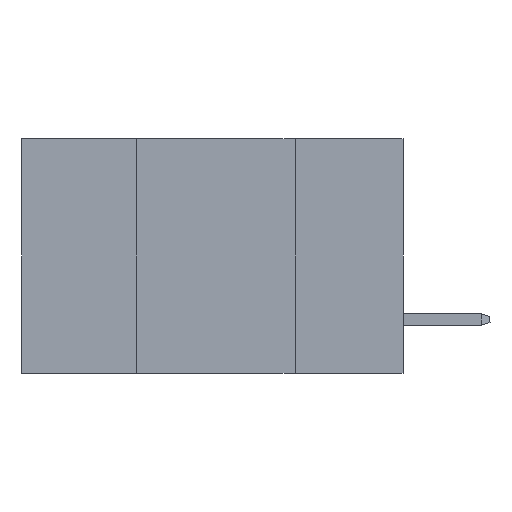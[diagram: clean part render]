
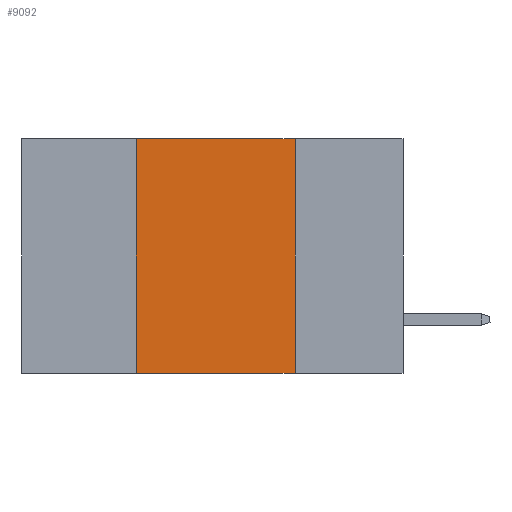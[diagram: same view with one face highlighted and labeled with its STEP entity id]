
A CAD part, left-side view. The second image highlights one B-rep face of the part: STEP entity #9092.
In plain terms, the highlighted planar face has unit normal (-1, 0, 0).
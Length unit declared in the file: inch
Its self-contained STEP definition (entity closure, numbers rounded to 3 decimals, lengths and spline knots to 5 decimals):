
#699 = VECTOR ( 'NONE', #11565, 39.37008 ) ;
#727 = EDGE_CURVE ( 'NONE', #1597, #11515, #3971, .T. ) ;
#1251 = EDGE_CURVE ( 'NONE', #15855, #9012, #5913, .T. ) ;
#1597 = VERTEX_POINT ( 'NONE', #13618 ) ;
#1926 = VECTOR ( 'NONE', #8427, 39.37008 ) ;
#2162 = PLANE ( 'NONE',  #11635 ) ;
#3344 = LINE ( 'NONE', #14631, #1926 ) ;
#3499 = DIRECTION ( 'NONE',  ( 0., 0., -1. ) ) ;
#3557 = DIRECTION ( 'NONE',  ( 0., 0., -1. ) ) ;
#3971 = LINE ( 'NONE', #5391, #8766 ) ;
#5391 = CARTESIAN_POINT ( 'NONE',  ( 0., 0.42, 0. ) ) ;
#5913 = LINE ( 'NONE', #5993, #7078 ) ;
#5993 = CARTESIAN_POINT ( 'NONE',  ( 0., 0.17, 0. ) ) ;
#6064 = FACE_OUTER_BOUND ( 'NONE', #6516, .T. ) ;
#6501 = CARTESIAN_POINT ( 'NONE',  ( 0., 0.6, 0. ) ) ;
#6516 = EDGE_LOOP ( 'NONE', ( #11091, #13093, #14889, #9731 ) ) ;
#7078 = VECTOR ( 'NONE', #3499, 39.37008 ) ;
#7250 = EDGE_CURVE ( 'NONE', #11515, #15855, #8907, .T. ) ;
#7310 = CARTESIAN_POINT ( 'NONE',  ( 0., 0.6, 0. ) ) ;
#8427 = DIRECTION ( 'NONE',  ( 0., -1., 0. ) ) ;
#8766 = VECTOR ( 'NONE', #9043, 39.37008 ) ;
#8907 = LINE ( 'NONE', #6501, #699 ) ;
#9012 = VERTEX_POINT ( 'NONE', #10788 ) ;
#9043 = DIRECTION ( 'NONE',  ( 0., 0., 1. ) ) ;
#9092 = ADVANCED_FACE ( 'NONE', ( #6064 ), #2162, .F. ) ;
#9423 = CARTESIAN_POINT ( 'NONE',  ( 0., 0.17, 0. ) ) ;
#9731 = ORIENTED_EDGE ( 'NONE', *, *, #14027, .T. ) ;
#10788 = CARTESIAN_POINT ( 'NONE',  ( 0., 0.17, -0.37 ) ) ;
#11091 = ORIENTED_EDGE ( 'NONE', *, *, #1251, .F. ) ;
#11515 = VERTEX_POINT ( 'NONE', #13627 ) ;
#11565 = DIRECTION ( 'NONE',  ( 0., -1., 0. ) ) ;
#11635 = AXIS2_PLACEMENT_3D ( 'NONE', #7310, #13700, #3557 ) ;
#13093 = ORIENTED_EDGE ( 'NONE', *, *, #7250, .F. ) ;
#13618 = CARTESIAN_POINT ( 'NONE',  ( 0., 0.42, -0.37 ) ) ;
#13627 = CARTESIAN_POINT ( 'NONE',  ( 0., 0.42, 0. ) ) ;
#13700 = DIRECTION ( 'NONE',  ( 1., 0., 0. ) ) ;
#14027 = EDGE_CURVE ( 'NONE', #1597, #9012, #3344, .T. ) ;
#14631 = CARTESIAN_POINT ( 'NONE',  ( 0., 0.6, -0.37 ) ) ;
#14889 = ORIENTED_EDGE ( 'NONE', *, *, #727, .F. ) ;
#15855 = VERTEX_POINT ( 'NONE', #9423 ) ;
